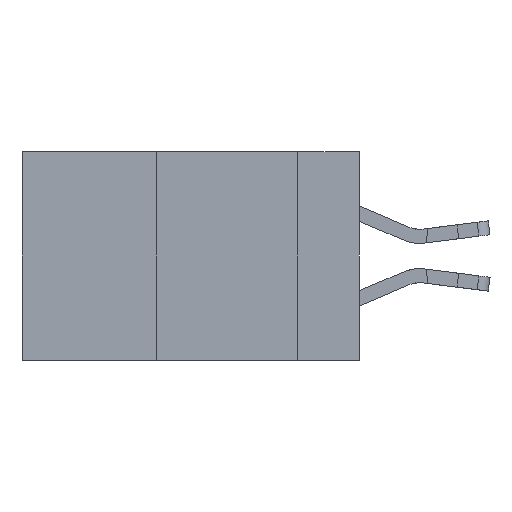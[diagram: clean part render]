
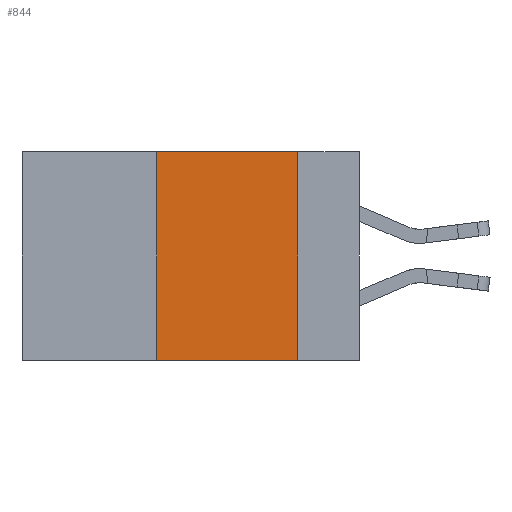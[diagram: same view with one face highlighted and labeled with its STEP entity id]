
A CAD part, left-side view. The second image highlights one B-rep face of the part: STEP entity #844.
In plain terms, the highlighted planar face has unit normal (-1, 0, 0).
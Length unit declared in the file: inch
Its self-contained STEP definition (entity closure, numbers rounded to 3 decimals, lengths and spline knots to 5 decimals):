
#844 = ADVANCED_FACE ( 'NONE', ( #22374 ), #6816, .F. ) ;
#970 = CARTESIAN_POINT ( 'NONE',  ( 0., 0.11, -0.37 ) ) ;
#1519 = ORIENTED_EDGE ( 'NONE', *, *, #17791, .T. ) ;
#1526 = CARTESIAN_POINT ( 'NONE',  ( 0., 0.6, 0. ) ) ;
#1747 = ORIENTED_EDGE ( 'NONE', *, *, #20880, .F. ) ;
#1766 = VERTEX_POINT ( 'NONE', #970 ) ;
#1841 = CARTESIAN_POINT ( 'NONE',  ( 0., 0.11, 0. ) ) ;
#2551 = ORIENTED_EDGE ( 'NONE', *, *, #16649, .F. ) ;
#2821 = EDGE_LOOP ( 'NONE', ( #17189, #1747, #2551, #1519 ) ) ;
#4060 = CARTESIAN_POINT ( 'NONE',  ( 0., 0.36, -0.37 ) ) ;
#4457 = DIRECTION ( 'NONE',  ( 0., 0., -1. ) ) ;
#4747 = LINE ( 'NONE', #6482, #8795 ) ;
#6012 = VECTOR ( 'NONE', #7496, 39.37008 ) ;
#6482 = CARTESIAN_POINT ( 'NONE',  ( 0., 0.6, 0. ) ) ;
#6550 = LINE ( 'NONE', #15996, #6012 ) ;
#6816 = PLANE ( 'NONE',  #19350 ) ;
#7364 = VECTOR ( 'NONE', #21217, 39.37008 ) ;
#7496 = DIRECTION ( 'NONE',  ( 0., -1., 0. ) ) ;
#7963 = VECTOR ( 'NONE', #22058, 39.37008 ) ;
#8211 = DIRECTION ( 'NONE',  ( 0., -1., 0. ) ) ;
#8795 = VECTOR ( 'NONE', #8211, 39.37008 ) ;
#10127 = CARTESIAN_POINT ( 'NONE',  ( 0., 0.11, 0. ) ) ;
#11541 = DIRECTION ( 'NONE',  ( 1., 0., 0. ) ) ;
#14557 = CARTESIAN_POINT ( 'NONE',  ( 0., 0.36, 0. ) ) ;
#15219 = VERTEX_POINT ( 'NONE', #16171 ) ;
#15509 = EDGE_CURVE ( 'NONE', #17165, #1766, #17101, .T. ) ;
#15996 = CARTESIAN_POINT ( 'NONE',  ( 0., 0.6, -0.37 ) ) ;
#16171 = CARTESIAN_POINT ( 'NONE',  ( 0., 0.36, 0. ) ) ;
#16524 = LINE ( 'NONE', #14557, #7364 ) ;
#16649 = EDGE_CURVE ( 'NONE', #20500, #15219, #16524, .T. ) ;
#17101 = LINE ( 'NONE', #10127, #7963 ) ;
#17165 = VERTEX_POINT ( 'NONE', #1841 ) ;
#17189 = ORIENTED_EDGE ( 'NONE', *, *, #15509, .F. ) ;
#17791 = EDGE_CURVE ( 'NONE', #20500, #1766, #6550, .T. ) ;
#19350 = AXIS2_PLACEMENT_3D ( 'NONE', #1526, #11541, #4457 ) ;
#20500 = VERTEX_POINT ( 'NONE', #4060 ) ;
#20880 = EDGE_CURVE ( 'NONE', #15219, #17165, #4747, .T. ) ;
#21217 = DIRECTION ( 'NONE',  ( 0., 0., 1. ) ) ;
#22058 = DIRECTION ( 'NONE',  ( 0., 0., -1. ) ) ;
#22374 = FACE_OUTER_BOUND ( 'NONE', #2821, .T. ) ;
